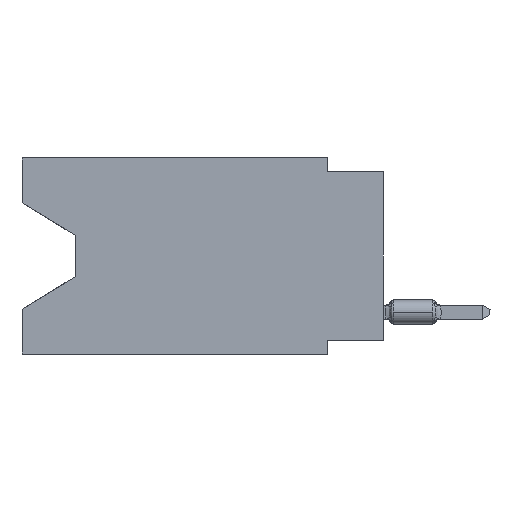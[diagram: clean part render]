
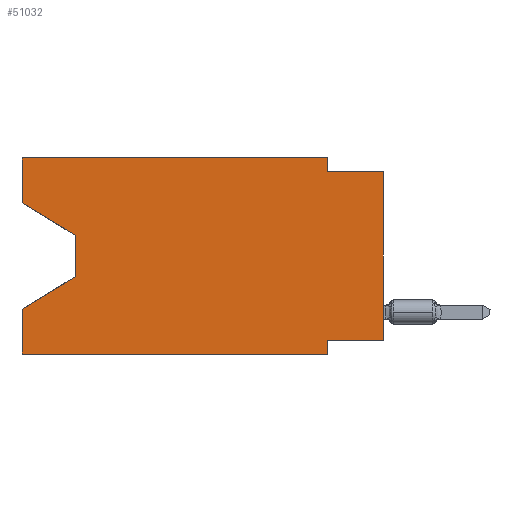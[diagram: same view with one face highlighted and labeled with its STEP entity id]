
A CAD part, left-side view. The second image highlights one B-rep face of the part: STEP entity #51032.
In plain terms, the highlighted planar face has unit normal (-1, 0, 0).
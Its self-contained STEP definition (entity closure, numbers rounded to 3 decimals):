
#540 = EDGE_CURVE ( 'NONE', #37164, #32028, #40694, .T. ) ;
#1332 = ORIENTED_EDGE ( 'NONE', *, *, #22691, .F. ) ;
#1851 = EDGE_CURVE ( 'NONE', #7223, #44363, #9928, .T. ) ;
#2729 = VERTEX_POINT ( 'NONE', #5124 ) ;
#3368 = ORIENTED_EDGE ( 'NONE', *, *, #25243, .T. ) ;
#3514 = VERTEX_POINT ( 'NONE', #6112 ) ;
#3564 = ORIENTED_EDGE ( 'NONE', *, *, #36994, .F. ) ;
#3662 = CARTESIAN_POINT ( 'NONE',  ( 0., 16.383, 0. ) ) ;
#5124 = CARTESIAN_POINT ( 'NONE',  ( 0., 16.383, -2.038 ) ) ;
#5943 = ORIENTED_EDGE ( 'NONE', *, *, #19601, .T. ) ;
#6112 = CARTESIAN_POINT ( 'NONE',  ( 0., 2.54, 0. ) ) ;
#6554 = EDGE_CURVE ( 'NONE', #2729, #37164, #9269, .T. ) ;
#7223 = VERTEX_POINT ( 'NONE', #59476 ) ;
#8317 = EDGE_CURVE ( 'NONE', #33036, #26755, #31355, .T. ) ;
#9269 = LINE ( 'NONE', #19209, #48581 ) ;
#9928 = LINE ( 'NONE', #57446, #32277 ) ;
#14291 = VECTOR ( 'NONE', #55297, 1000. ) ;
#14524 = LINE ( 'NONE', #38407, #44470 ) ;
#14840 = DIRECTION ( 'NONE',  ( 0., 0., 1. ) ) ;
#15532 = CARTESIAN_POINT ( 'NONE',  ( 0., 2.54, 0. ) ) ;
#15536 = VERTEX_POINT ( 'NONE', #41288 ) ;
#16947 = EDGE_CURVE ( 'NONE', #7223, #21642, #20649, .T. ) ;
#17673 = DIRECTION ( 'NONE',  ( 0., 0., -1. ) ) ;
#17991 = CARTESIAN_POINT ( 'NONE',  ( 0., 13.97, -5.385 ) ) ;
#19209 = CARTESIAN_POINT ( 'NONE',  ( 0., 16.383, -2.038 ) ) ;
#19601 = EDGE_CURVE ( 'NONE', #32028, #44363, #42441, .T. ) ;
#20649 = LINE ( 'NONE', #34936, #52677 ) ;
#21064 = LINE ( 'NONE', #15532, #21674 ) ;
#21486 = DIRECTION ( 'NONE',  ( 0., -1., 0. ) ) ;
#21642 = VERTEX_POINT ( 'NONE', #28912 ) ;
#21674 = VECTOR ( 'NONE', #39999, 1000. ) ;
#22368 = CARTESIAN_POINT ( 'NONE',  ( 0., 13.97, -3.505 ) ) ;
#22691 = EDGE_CURVE ( 'NONE', #15536, #37428, #61238, .T. ) ;
#22974 = CARTESIAN_POINT ( 'NONE',  ( 0., 0., -8.255 ) ) ;
#24074 = CARTESIAN_POINT ( 'NONE',  ( 0., 13.97, -3.505 ) ) ;
#24913 = AXIS2_PLACEMENT_3D ( 'NONE', #3662, #31934, #17673 ) ;
#25243 = EDGE_CURVE ( 'NONE', #33036, #37428, #34009, .T. ) ;
#25536 = ORIENTED_EDGE ( 'NONE', *, *, #1851, .F. ) ;
#26145 = CARTESIAN_POINT ( 'NONE',  ( 0., 16.383, 0. ) ) ;
#26203 = LINE ( 'NONE', #27122, #58509 ) ;
#26303 = VERTEX_POINT ( 'NONE', #36897 ) ;
#26755 = VERTEX_POINT ( 'NONE', #41819 ) ;
#27122 = CARTESIAN_POINT ( 'NONE',  ( 0., 2.54, -8.89 ) ) ;
#27126 = VECTOR ( 'NONE', #34624, 1000. ) ;
#28295 = CARTESIAN_POINT ( 'NONE',  ( 0., 0., -0.635 ) ) ;
#28912 = CARTESIAN_POINT ( 'NONE',  ( 0., 2.54, -8.89 ) ) ;
#30269 = VECTOR ( 'NONE', #32022, 1000. ) ;
#30496 = LINE ( 'NONE', #26145, #58802 ) ;
#31355 = LINE ( 'NONE', #22974, #58490 ) ;
#31934 = DIRECTION ( 'NONE',  ( 1., 0., 0. ) ) ;
#32022 = DIRECTION ( 'NONE',  ( 0., -1., 0. ) ) ;
#32028 = VERTEX_POINT ( 'NONE', #17991 ) ;
#32185 = EDGE_LOOP ( 'NONE', ( #60361, #36248, #5943, #25536, #44611, #51247, #58591, #3368, #1332, #59373, #3564, #48814 ) ) ;
#32277 = VECTOR ( 'NONE', #37568, 1000. ) ;
#32763 = CARTESIAN_POINT ( 'NONE',  ( 0., 16.383, -6.852 ) ) ;
#33036 = VERTEX_POINT ( 'NONE', #33261 ) ;
#33261 = CARTESIAN_POINT ( 'NONE',  ( 0., 0., -8.255 ) ) ;
#34009 = LINE ( 'NONE', #49203, #27126 ) ;
#34624 = DIRECTION ( 'NONE',  ( 0., 0., 1. ) ) ;
#34936 = CARTESIAN_POINT ( 'NONE',  ( 0., 16.383, -8.89 ) ) ;
#36006 = DIRECTION ( 'NONE',  ( 0., 1., 0. ) ) ;
#36248 = ORIENTED_EDGE ( 'NONE', *, *, #540, .T. ) ;
#36897 = CARTESIAN_POINT ( 'NONE',  ( 0., 16.383, 0. ) ) ;
#36994 = EDGE_CURVE ( 'NONE', #26303, #3514, #30496, .T. ) ;
#37164 = VERTEX_POINT ( 'NONE', #24074 ) ;
#37428 = VERTEX_POINT ( 'NONE', #57557 ) ;
#37568 = DIRECTION ( 'NONE',  ( 0., 0., 1. ) ) ;
#38407 = CARTESIAN_POINT ( 'NONE',  ( 0., 16.383, 0. ) ) ;
#39999 = DIRECTION ( 'NONE',  ( 0., 0., -1. ) ) ;
#40087 = EDGE_CURVE ( 'NONE', #2729, #26303, #14524, .T. ) ;
#40694 = LINE ( 'NONE', #22368, #14291 ) ;
#41288 = CARTESIAN_POINT ( 'NONE',  ( 0., 2.54, -0.635 ) ) ;
#41819 = CARTESIAN_POINT ( 'NONE',  ( 0., 2.54, -8.255 ) ) ;
#42441 = LINE ( 'NONE', #51761, #43807 ) ;
#43807 = VECTOR ( 'NONE', #46792, 1000. ) ;
#44363 = VERTEX_POINT ( 'NONE', #32763 ) ;
#44470 = VECTOR ( 'NONE', #14840, 1000. ) ;
#44611 = ORIENTED_EDGE ( 'NONE', *, *, #16947, .T. ) ;
#46792 = DIRECTION ( 'NONE',  ( 0., 0.855, -0.519 ) ) ;
#47138 = FACE_OUTER_BOUND ( 'NONE', #32185, .T. ) ;
#48581 = VECTOR ( 'NONE', #60844, 1000. ) ;
#48814 = ORIENTED_EDGE ( 'NONE', *, *, #40087, .F. ) ;
#49203 = CARTESIAN_POINT ( 'NONE',  ( 0., 0., 0. ) ) ;
#50106 = DIRECTION ( 'NONE',  ( 0., 0., -1. ) ) ;
#51032 = ADVANCED_FACE ( 'NONE', ( #47138 ), #56487, .F. ) ;
#51247 = ORIENTED_EDGE ( 'NONE', *, *, #59130, .F. ) ;
#51761 = CARTESIAN_POINT ( 'NONE',  ( 0., 13.97, -5.385 ) ) ;
#52677 = VECTOR ( 'NONE', #53882, 1000. ) ;
#53882 = DIRECTION ( 'NONE',  ( 0., -1., 0. ) ) ;
#55297 = DIRECTION ( 'NONE',  ( 0., 0., -1. ) ) ;
#56487 = PLANE ( 'NONE',  #24913 ) ;
#56964 = EDGE_CURVE ( 'NONE', #3514, #15536, #21064, .T. ) ;
#57446 = CARTESIAN_POINT ( 'NONE',  ( 0., 16.383, 0. ) ) ;
#57557 = CARTESIAN_POINT ( 'NONE',  ( 0., 0., -0.635 ) ) ;
#58490 = VECTOR ( 'NONE', #36006, 1000. ) ;
#58509 = VECTOR ( 'NONE', #50106, 1000. ) ;
#58591 = ORIENTED_EDGE ( 'NONE', *, *, #8317, .F. ) ;
#58802 = VECTOR ( 'NONE', #21486, 1000. ) ;
#59130 = EDGE_CURVE ( 'NONE', #26755, #21642, #26203, .T. ) ;
#59373 = ORIENTED_EDGE ( 'NONE', *, *, #56964, .F. ) ;
#59476 = CARTESIAN_POINT ( 'NONE',  ( 0., 16.383, -8.89 ) ) ;
#60361 = ORIENTED_EDGE ( 'NONE', *, *, #6554, .T. ) ;
#60844 = DIRECTION ( 'NONE',  ( 0., -0.855, -0.519 ) ) ;
#61238 = LINE ( 'NONE', #28295, #30269 ) ;
